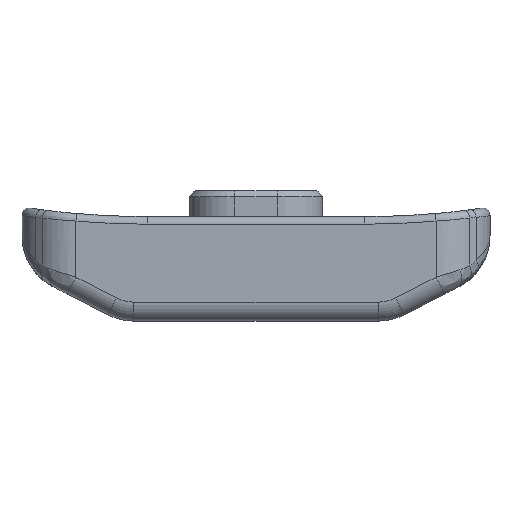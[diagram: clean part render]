
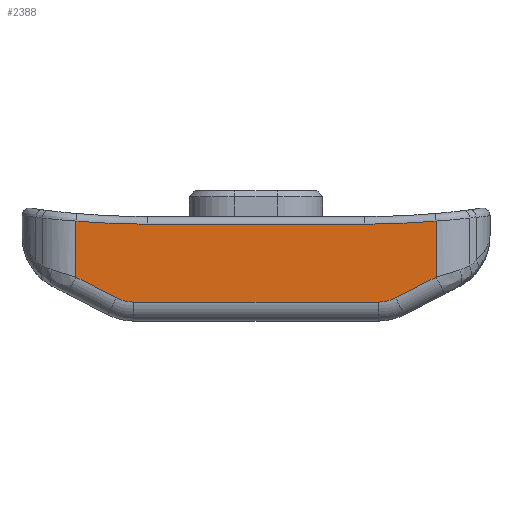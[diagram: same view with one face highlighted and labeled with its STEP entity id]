
A CAD part, front view. The second image highlights one B-rep face of the part: STEP entity #2388.
In plain terms, the highlighted planar face has unit normal (0, -1, 0).
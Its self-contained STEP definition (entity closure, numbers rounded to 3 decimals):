
#233=CIRCLE('',#2604,2.);
#237=CIRCLE('',#2613,43.691);
#238=CIRCLE('',#2614,43.691);
#239=CIRCLE('',#2615,2.);
#412=FACE_OUTER_BOUND('',#579,.T.);
#579=EDGE_LOOP('',(#1821,#1822,#1823,#1824,#1825,#1826,#1827,#1828,#1829,
#1830));
#784=LINE('',#3877,#932);
#785=LINE('',#3881,#933);
#786=LINE('',#3883,#934);
#787=LINE('',#3887,#935);
#788=LINE('',#3891,#936);
#789=LINE('',#3893,#937);
#932=VECTOR('',#3120,10.);
#933=VECTOR('',#3125,10.);
#934=VECTOR('',#3126,10.);
#935=VECTOR('',#3129,10.);
#936=VECTOR('',#3132,10.);
#937=VECTOR('',#3133,10.);
#1068=VERTEX_POINT('',#3852);
#1071=VERTEX_POINT('',#3857);
#1076=VERTEX_POINT('',#3876);
#1077=VERTEX_POINT('',#3880);
#1078=VERTEX_POINT('',#3882);
#1079=VERTEX_POINT('',#3884);
#1080=VERTEX_POINT('',#3886);
#1081=VERTEX_POINT('',#3888);
#1082=VERTEX_POINT('',#3890);
#1083=VERTEX_POINT('',#3892);
#1332=EDGE_CURVE('',#1071,#1068,#233,.T.);
#1341=EDGE_CURVE('',#1068,#1076,#784,.T.);
#1343=EDGE_CURVE('',#1077,#1071,#785,.T.);
#1344=EDGE_CURVE('',#1078,#1077,#786,.T.);
#1345=EDGE_CURVE('',#1079,#1078,#237,.T.);
#1346=EDGE_CURVE('',#1080,#1079,#787,.T.);
#1347=EDGE_CURVE('',#1081,#1080,#238,.T.);
#1348=EDGE_CURVE('',#1082,#1081,#788,.T.);
#1349=EDGE_CURVE('',#1083,#1082,#789,.T.);
#1350=EDGE_CURVE('',#1076,#1083,#239,.T.);
#1821=ORIENTED_EDGE('',*,*,#1332,.F.);
#1822=ORIENTED_EDGE('',*,*,#1343,.F.);
#1823=ORIENTED_EDGE('',*,*,#1344,.F.);
#1824=ORIENTED_EDGE('',*,*,#1345,.F.);
#1825=ORIENTED_EDGE('',*,*,#1346,.F.);
#1826=ORIENTED_EDGE('',*,*,#1347,.F.);
#1827=ORIENTED_EDGE('',*,*,#1348,.F.);
#1828=ORIENTED_EDGE('',*,*,#1349,.F.);
#1829=ORIENTED_EDGE('',*,*,#1350,.F.);
#1830=ORIENTED_EDGE('',*,*,#1341,.F.);
#2314=PLANE('',#2612);
#2388=ADVANCED_FACE('',(#412),#2314,.T.);
#2604=AXIS2_PLACEMENT_3D('',#3859,#3100,#3101);
#2612=AXIS2_PLACEMENT_3D('',#3879,#3123,#3124);
#2613=AXIS2_PLACEMENT_3D('',#3885,#3127,#3128);
#2614=AXIS2_PLACEMENT_3D('',#3889,#3130,#3131);
#2615=AXIS2_PLACEMENT_3D('',#3894,#3134,#3135);
#3100=DIRECTION('center_axis',(0.,1.,0.));
#3101=DIRECTION('ref_axis',(0.235,0.,-0.972));
#3120=DIRECTION('',(-1.,0.,0.));
#3123=DIRECTION('center_axis',(0.,-1.,0.));
#3124=DIRECTION('ref_axis',(0.,0.,-1.));
#3125=DIRECTION('',(-0.889,0.,-0.457));
#3126=DIRECTION('',(0.,0.,-1.));
#3127=DIRECTION('center_axis',(0.,-1.,0.));
#3128=DIRECTION('ref_axis',(0.043,0.,-0.999));
#3129=DIRECTION('',(1.,0.,0.));
#3130=DIRECTION('center_axis',(0.,-1.,0.));
#3131=DIRECTION('ref_axis',(-0.043,0.,-0.999));
#3132=DIRECTION('',(0.,0.,1.));
#3133=DIRECTION('',(-0.889,0.,0.457));
#3134=DIRECTION('center_axis',(0.,1.,0.));
#3135=DIRECTION('ref_axis',(-0.235,0.,-0.972));
#3852=CARTESIAN_POINT('',(-33.579,-15.5,-7.3));
#3857=CARTESIAN_POINT('',(-32.665,-15.5,-7.079));
#3859=CARTESIAN_POINT('Origin',(-33.579,-15.5,-5.3));
#3876=CARTESIAN_POINT('',(-46.421,-15.5,-7.3));
#3877=CARTESIAN_POINT('',(-46.25,-15.5,-7.3));
#3879=CARTESIAN_POINT('Origin',(-40.,-15.5,-4.7));
#3880=CARTESIAN_POINT('',(-30.536,-15.5,-5.985));
#3881=CARTESIAN_POINT('',(-35.406,-15.5,-8.487));
#3882=CARTESIAN_POINT('',(-30.536,-15.5,-3.039));
#3883=CARTESIAN_POINT('',(-30.536,-15.5,-4.225));
#3884=CARTESIAN_POINT('',(-34.287,-15.5,-3.2));
#3885=CARTESIAN_POINT('Origin',(-34.287,-15.5,40.491));
#3886=CARTESIAN_POINT('',(-45.713,-15.5,-3.2));
#3887=CARTESIAN_POINT('',(-40.,-15.5,-3.2));
#3888=CARTESIAN_POINT('',(-49.464,-15.5,-3.039));
#3889=CARTESIAN_POINT('Origin',(-45.713,-15.5,40.491));
#3890=CARTESIAN_POINT('',(-49.464,-15.5,-5.985));
#3891=CARTESIAN_POINT('',(-49.464,-15.5,-4.225));
#3892=CARTESIAN_POINT('',(-47.335,-15.5,-7.079));
#3893=CARTESIAN_POINT('',(-47.271,-15.5,-7.112));
#3894=CARTESIAN_POINT('Origin',(-46.421,-15.5,-5.3));
